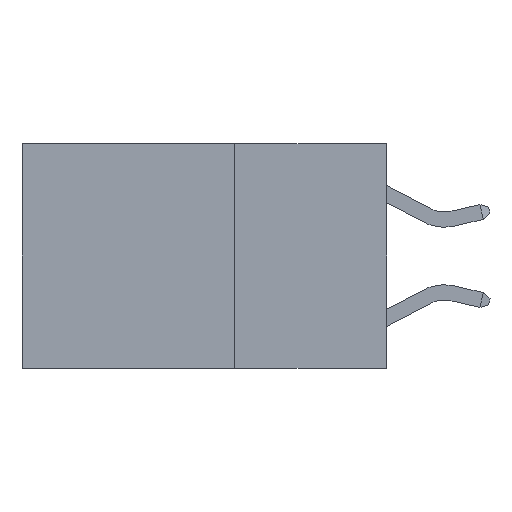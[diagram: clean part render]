
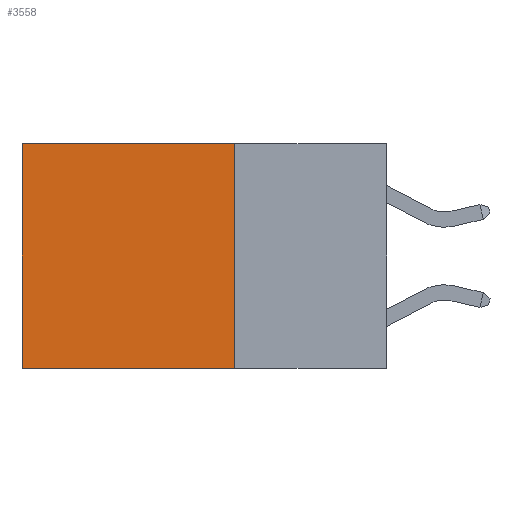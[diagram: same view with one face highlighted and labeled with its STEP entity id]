
A CAD part, left-side view. The second image highlights one B-rep face of the part: STEP entity #3558.
In plain terms, the highlighted planar face has unit normal (-1, 0, 0).
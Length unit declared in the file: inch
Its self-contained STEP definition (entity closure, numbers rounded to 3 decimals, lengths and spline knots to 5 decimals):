
#377 = VERTEX_POINT ( 'NONE', #11630 ) ;
#906 = VERTEX_POINT ( 'NONE', #12043 ) ;
#1168 = VERTEX_POINT ( 'NONE', #3957 ) ;
#1346 = CARTESIAN_POINT ( 'NONE',  ( 0.2625, 0.6, 0. ) ) ;
#1853 = DIRECTION ( 'NONE',  ( 0., 1., 0. ) ) ;
#1945 = VECTOR ( 'NONE', #6603, 39.37008 ) ;
#3242 = LINE ( 'NONE', #10536, #5859 ) ;
#3425 = EDGE_LOOP ( 'NONE', ( #6934, #7689, #4657, #5488 ) ) ;
#3511 = AXIS2_PLACEMENT_3D ( 'NONE', #11233, #12148, #6538 ) ;
#3558 = ADVANCED_FACE ( 'NONE', ( #3742 ), #4602, .F. ) ;
#3742 = FACE_OUTER_BOUND ( 'NONE', #3425, .T. ) ;
#3957 = CARTESIAN_POINT ( 'NONE',  ( 0.2625, 0.6, 0. ) ) ;
#4058 = CARTESIAN_POINT ( 'NONE',  ( 0.2625, 0.25, 0. ) ) ;
#4602 = PLANE ( 'NONE',  #3511 ) ;
#4657 = ORIENTED_EDGE ( 'NONE', *, *, #8361, .F. ) ;
#4683 = CARTESIAN_POINT ( 'NONE',  ( 0.2625, 0.25, 0. ) ) ;
#4859 = DIRECTION ( 'NONE',  ( 0., 1., 0. ) ) ;
#5222 = VECTOR ( 'NONE', #10017, 39.37008 ) ;
#5488 = ORIENTED_EDGE ( 'NONE', *, *, #12417, .T. ) ;
#5859 = VECTOR ( 'NONE', #4859, 39.37008 ) ;
#6170 = EDGE_CURVE ( 'NONE', #1168, #377, #7444, .T. ) ;
#6538 = DIRECTION ( 'NONE',  ( 0., 0., -1. ) ) ;
#6603 = DIRECTION ( 'NONE',  ( 0., 0., -1. ) ) ;
#6655 = VERTEX_POINT ( 'NONE', #4058 ) ;
#6833 = LINE ( 'NONE', #4683, #1945 ) ;
#6934 = ORIENTED_EDGE ( 'NONE', *, *, #6170, .T. ) ;
#7444 = LINE ( 'NONE', #1346, #5222 ) ;
#7689 = ORIENTED_EDGE ( 'NONE', *, *, #8454, .F. ) ;
#8203 = LINE ( 'NONE', #8673, #8505 ) ;
#8361 = EDGE_CURVE ( 'NONE', #6655, #906, #6833, .T. ) ;
#8454 = EDGE_CURVE ( 'NONE', #906, #377, #8203, .T. ) ;
#8505 = VECTOR ( 'NONE', #1853, 39.37008 ) ;
#8673 = CARTESIAN_POINT ( 'NONE',  ( 0.2625, 0.25, -0.37 ) ) ;
#10017 = DIRECTION ( 'NONE',  ( 0., 0., -1. ) ) ;
#10536 = CARTESIAN_POINT ( 'NONE',  ( 0.2625, 0.25, 0. ) ) ;
#11233 = CARTESIAN_POINT ( 'NONE',  ( 0.2625, 0.25, 0. ) ) ;
#11630 = CARTESIAN_POINT ( 'NONE',  ( 0.2625, 0.6, -0.37 ) ) ;
#12043 = CARTESIAN_POINT ( 'NONE',  ( 0.2625, 0.25, -0.37 ) ) ;
#12148 = DIRECTION ( 'NONE',  ( 1., 0., 0. ) ) ;
#12417 = EDGE_CURVE ( 'NONE', #6655, #1168, #3242, .T. ) ;
